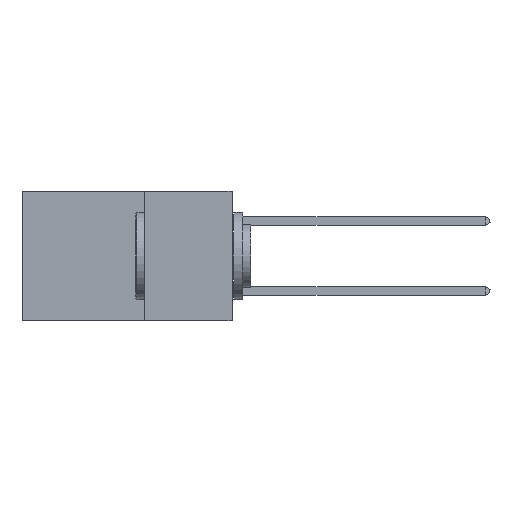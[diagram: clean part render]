
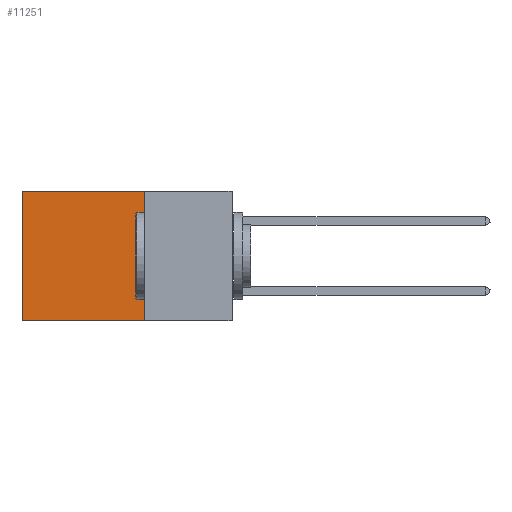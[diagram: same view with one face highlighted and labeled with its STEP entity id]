
A CAD part, left-side view. The second image highlights one B-rep face of the part: STEP entity #11251.
In plain terms, the highlighted planar face has unit normal (-1, 0, 0).
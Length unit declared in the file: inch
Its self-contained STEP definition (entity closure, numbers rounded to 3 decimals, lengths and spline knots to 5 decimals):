
#165 = DIRECTION ( 'NONE',  ( 0., 1., 0. ) ) ;
#582 = FACE_OUTER_BOUND ( 'NONE', #2350, .T. ) ;
#955 = LINE ( 'NONE', #12328, #5261 ) ;
#1236 = DIRECTION ( 'NONE',  ( 1., 0., 0. ) ) ;
#2350 = EDGE_LOOP ( 'NONE', ( #10239, #19111, #4972, #22579 ) ) ;
#3170 = VERTEX_POINT ( 'NONE', #15396 ) ;
#4375 = CARTESIAN_POINT ( 'NONE',  ( 0.2875, 0.6, 0. ) ) ;
#4972 = ORIENTED_EDGE ( 'NONE', *, *, #14957, .F. ) ;
#5261 = VECTOR ( 'NONE', #14021, 39.37008 ) ;
#5606 = LINE ( 'NONE', #10887, #19315 ) ;
#5661 = AXIS2_PLACEMENT_3D ( 'NONE', #18633, #1236, #13513 ) ;
#7251 = LINE ( 'NONE', #17059, #21945 ) ;
#7555 = CARTESIAN_POINT ( 'NONE',  ( 0.2875, 0.6, 0. ) ) ;
#9071 = VERTEX_POINT ( 'NONE', #10786 ) ;
#9376 = EDGE_CURVE ( 'NONE', #17422, #19286, #7251, .T. ) ;
#9446 = LINE ( 'NONE', #7555, #18547 ) ;
#10239 = ORIENTED_EDGE ( 'NONE', *, *, #21618, .T. ) ;
#10786 = CARTESIAN_POINT ( 'NONE',  ( 0.2875, 0.25, -0.37 ) ) ;
#10887 = CARTESIAN_POINT ( 'NONE',  ( 0.2875, 0.25, -0.37 ) ) ;
#11251 = ADVANCED_FACE ( 'NONE', ( #582 ), #11825, .F. ) ;
#11825 = PLANE ( 'NONE',  #5661 ) ;
#12328 = CARTESIAN_POINT ( 'NONE',  ( 0.2875, 0.25, 0. ) ) ;
#13513 = DIRECTION ( 'NONE',  ( 0., 0., -1. ) ) ;
#13603 = DIRECTION ( 'NONE',  ( 0., 1., 0. ) ) ;
#14021 = DIRECTION ( 'NONE',  ( 0., 0., -1. ) ) ;
#14352 = DIRECTION ( 'NONE',  ( 0., 0., -1. ) ) ;
#14957 = EDGE_CURVE ( 'NONE', #17422, #9071, #955, .T. ) ;
#15396 = CARTESIAN_POINT ( 'NONE',  ( 0.2875, 0.6, -0.37 ) ) ;
#17059 = CARTESIAN_POINT ( 'NONE',  ( 0.2875, 0.25, 0. ) ) ;
#17422 = VERTEX_POINT ( 'NONE', #21909 ) ;
#18547 = VECTOR ( 'NONE', #14352, 39.37008 ) ;
#18633 = CARTESIAN_POINT ( 'NONE',  ( 0.2875, 0.25, 0. ) ) ;
#19111 = ORIENTED_EDGE ( 'NONE', *, *, #22253, .F. ) ;
#19286 = VERTEX_POINT ( 'NONE', #4375 ) ;
#19315 = VECTOR ( 'NONE', #165, 39.37008 ) ;
#21618 = EDGE_CURVE ( 'NONE', #19286, #3170, #9446, .T. ) ;
#21909 = CARTESIAN_POINT ( 'NONE',  ( 0.2875, 0.25, 0. ) ) ;
#21945 = VECTOR ( 'NONE', #13603, 39.37008 ) ;
#22253 = EDGE_CURVE ( 'NONE', #9071, #3170, #5606, .T. ) ;
#22579 = ORIENTED_EDGE ( 'NONE', *, *, #9376, .T. ) ;
